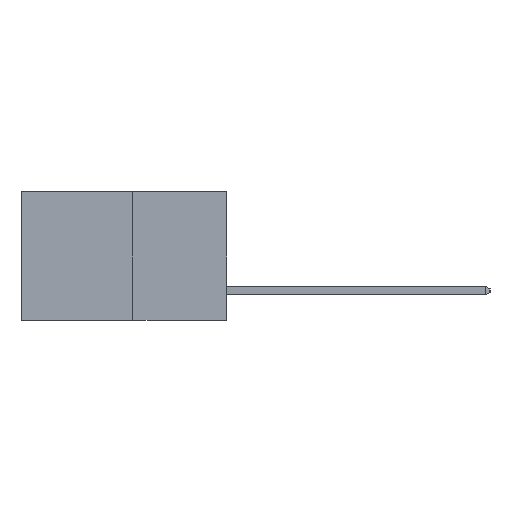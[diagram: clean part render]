
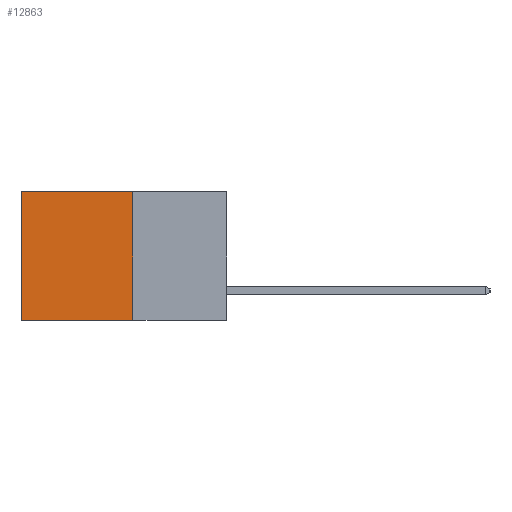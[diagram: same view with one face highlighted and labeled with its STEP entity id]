
A CAD part, left-side view. The second image highlights one B-rep face of the part: STEP entity #12863.
In plain terms, the highlighted planar face has unit normal (-1, 0, 0).
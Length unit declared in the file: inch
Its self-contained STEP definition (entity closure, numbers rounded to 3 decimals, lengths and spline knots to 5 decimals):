
#129 = VERTEX_POINT ( 'NONE', #16142 ) ;
#805 = VERTEX_POINT ( 'NONE', #21763 ) ;
#3892 = CARTESIAN_POINT ( 'NONE',  ( 0.277, 0.59, 0. ) ) ;
#4479 = CARTESIAN_POINT ( 'NONE',  ( 0.277, 0.59, -0.37 ) ) ;
#6123 = DIRECTION ( 'NONE',  ( 0., 1., 0. ) ) ;
#6144 = ORIENTED_EDGE ( 'NONE', *, *, #20615, .T. ) ;
#6869 = CARTESIAN_POINT ( 'NONE',  ( 0.277, 0.27, -0.37 ) ) ;
#8691 = DIRECTION ( 'NONE',  ( 0., 0., -1. ) ) ;
#9766 = DIRECTION ( 'NONE',  ( 0., 0., -1. ) ) ;
#9808 = EDGE_CURVE ( 'NONE', #13874, #11434, #15958, .T. ) ;
#10960 = VECTOR ( 'NONE', #21906, 39.37008 ) ;
#11339 = FACE_OUTER_BOUND ( 'NONE', #16985, .T. ) ;
#11434 = VERTEX_POINT ( 'NONE', #13553 ) ;
#12682 = ORIENTED_EDGE ( 'NONE', *, *, #19598, .F. ) ;
#12863 = ADVANCED_FACE ( 'NONE', ( #11339 ), #14044, .F. ) ;
#13553 = CARTESIAN_POINT ( 'NONE',  ( 0.277, 0.59, -0.37 ) ) ;
#13874 = VERTEX_POINT ( 'NONE', #3892 ) ;
#14044 = PLANE ( 'NONE',  #14142 ) ;
#14056 = VECTOR ( 'NONE', #6123, 39.37008 ) ;
#14142 = AXIS2_PLACEMENT_3D ( 'NONE', #6869, #19426, #8691 ) ;
#14605 = ORIENTED_EDGE ( 'NONE', *, *, #20516, .F. ) ;
#14621 = LINE ( 'NONE', #16927, #14056 ) ;
#15376 = ORIENTED_EDGE ( 'NONE', *, *, #9808, .T. ) ;
#15728 = LINE ( 'NONE', #16616, #10960 ) ;
#15958 = LINE ( 'NONE', #4479, #20138 ) ;
#16142 = CARTESIAN_POINT ( 'NONE',  ( 0.277, 0.27, -0.37 ) ) ;
#16616 = CARTESIAN_POINT ( 'NONE',  ( 0.277, 0.27, -0.37 ) ) ;
#16927 = CARTESIAN_POINT ( 'NONE',  ( 0.277, 0.27, 0. ) ) ;
#16985 = EDGE_LOOP ( 'NONE', ( #15376, #12682, #14605, #6144 ) ) ;
#17345 = DIRECTION ( 'NONE',  ( 0., 1., 0. ) ) ;
#18052 = LINE ( 'NONE', #22523, #21590 ) ;
#19426 = DIRECTION ( 'NONE',  ( 1., 0., 0. ) ) ;
#19598 = EDGE_CURVE ( 'NONE', #129, #11434, #18052, .T. ) ;
#20138 = VECTOR ( 'NONE', #9766, 39.37008 ) ;
#20516 = EDGE_CURVE ( 'NONE', #805, #129, #15728, .T. ) ;
#20615 = EDGE_CURVE ( 'NONE', #805, #13874, #14621, .T. ) ;
#21590 = VECTOR ( 'NONE', #17345, 39.37008 ) ;
#21763 = CARTESIAN_POINT ( 'NONE',  ( 0.277, 0.27, 0. ) ) ;
#21906 = DIRECTION ( 'NONE',  ( 0., 0., -1. ) ) ;
#22523 = CARTESIAN_POINT ( 'NONE',  ( 0.277, 0.27, -0.37 ) ) ;
